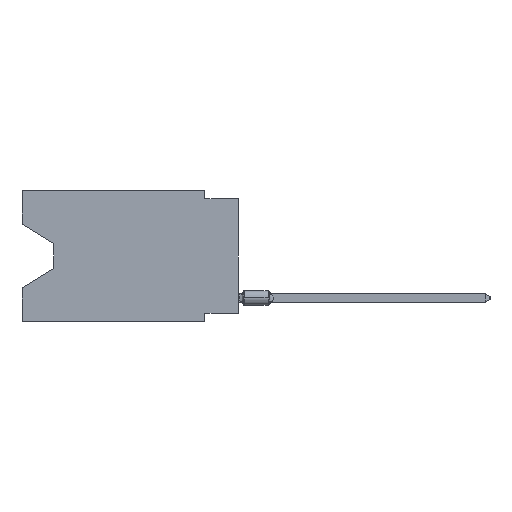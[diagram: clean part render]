
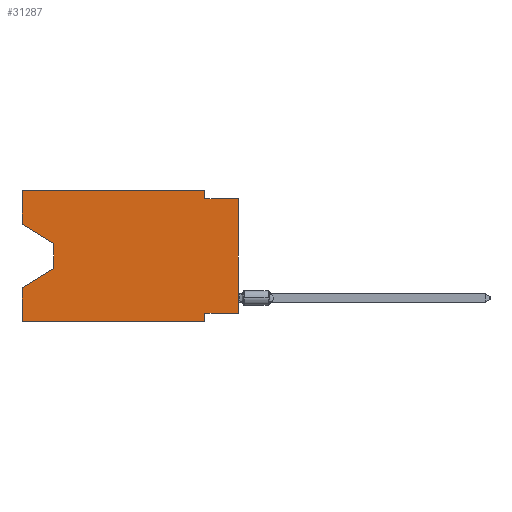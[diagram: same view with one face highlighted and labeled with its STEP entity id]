
A CAD part, left-side view. The second image highlights one B-rep face of the part: STEP entity #31287.
In plain terms, the highlighted planar face has unit normal (-1, 0, 0).
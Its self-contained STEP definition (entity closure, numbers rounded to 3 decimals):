
#125 = DIRECTION ( 'NONE',  ( 0., -1., 0. ) ) ;
#308 = LINE ( 'NONE', #8525, #14519 ) ;
#817 = EDGE_LOOP ( 'NONE', ( #17365, #26745, #19887, #10592, #1843, #28279, #2164, #14167, #22640, #7682, #24752, #28657 ) ) ;
#1843 = ORIENTED_EDGE ( 'NONE', *, *, #13814, .T. ) ;
#2164 = ORIENTED_EDGE ( 'NONE', *, *, #15014, .F. ) ;
#2192 = PLANE ( 'NONE',  #24027 ) ;
#2262 = DIRECTION ( 'NONE',  ( 0., 0.855, -0.519 ) ) ;
#2715 = CARTESIAN_POINT ( 'NONE',  ( 0., 16.383, -2.546 ) ) ;
#2917 = CARTESIAN_POINT ( 'NONE',  ( 0., 13.97, -4.013 ) ) ;
#3113 = VECTOR ( 'NONE', #27733, 1000. ) ;
#3210 = VERTEX_POINT ( 'NONE', #22563 ) ;
#3453 = DIRECTION ( 'NONE',  ( 0., 0., 1. ) ) ;
#4408 = DIRECTION ( 'NONE',  ( 1., 0., 0. ) ) ;
#4521 = CARTESIAN_POINT ( 'NONE',  ( 0., 2.54, -9.906 ) ) ;
#4547 = VERTEX_POINT ( 'NONE', #11504 ) ;
#6023 = VECTOR ( 'NONE', #19433, 1000. ) ;
#6717 = CARTESIAN_POINT ( 'NONE',  ( 0., 16.383, 0. ) ) ;
#7682 = ORIENTED_EDGE ( 'NONE', *, *, #28878, .F. ) ;
#7961 = CARTESIAN_POINT ( 'NONE',  ( 0., 16.383, -7.36 ) ) ;
#7990 = DIRECTION ( 'NONE',  ( 0., -1., 0. ) ) ;
#8167 = CARTESIAN_POINT ( 'NONE',  ( 0., 16.383, 0. ) ) ;
#8381 = LINE ( 'NONE', #19531, #22741 ) ;
#8525 = CARTESIAN_POINT ( 'NONE',  ( 0., 0., -0.635 ) ) ;
#8917 = DIRECTION ( 'NONE',  ( 0., 0., 1. ) ) ;
#10171 = LINE ( 'NONE', #21320, #15513 ) ;
#10301 = CARTESIAN_POINT ( 'NONE',  ( 0., 2.54, 0. ) ) ;
#10577 = DIRECTION ( 'NONE',  ( 0., 0., -1. ) ) ;
#10592 = ORIENTED_EDGE ( 'NONE', *, *, #18751, .F. ) ;
#10702 = DIRECTION ( 'NONE',  ( 0., 0., -1. ) ) ;
#11213 = LINE ( 'NONE', #4521, #6023 ) ;
#11255 = VERTEX_POINT ( 'NONE', #15968 ) ;
#11345 = CARTESIAN_POINT ( 'NONE',  ( 0., 0., -0.635 ) ) ;
#11444 = EDGE_CURVE ( 'NONE', #25396, #13808, #308, .T. ) ;
#11504 = CARTESIAN_POINT ( 'NONE',  ( 0., 13.97, -5.893 ) ) ;
#12002 = VECTOR ( 'NONE', #20411, 1000. ) ;
#13296 = EDGE_CURVE ( 'NONE', #3210, #30703, #11213, .T. ) ;
#13596 = LINE ( 'NONE', #27284, #18407 ) ;
#13808 = VERTEX_POINT ( 'NONE', #11345 ) ;
#13814 = EDGE_CURVE ( 'NONE', #27482, #30703, #17544, .T. ) ;
#14167 = ORIENTED_EDGE ( 'NONE', *, *, #35655, .T. ) ;
#14519 = VECTOR ( 'NONE', #125, 1000. ) ;
#14592 = LINE ( 'NONE', #15304, #20097 ) ;
#14639 = DIRECTION ( 'NONE',  ( 0., -1., 0. ) ) ;
#15014 = EDGE_CURVE ( 'NONE', #17722, #3210, #14592, .T. ) ;
#15304 = CARTESIAN_POINT ( 'NONE',  ( 0., 0., -9.271 ) ) ;
#15513 = VECTOR ( 'NONE', #10702, 1000. ) ;
#15968 = CARTESIAN_POINT ( 'NONE',  ( 0., 16.383, 0. ) ) ;
#16700 = CARTESIAN_POINT ( 'NONE',  ( 0., 13.97, -4.013 ) ) ;
#16781 = VECTOR ( 'NONE', #27947, 1000. ) ;
#16807 = VECTOR ( 'NONE', #7990, 1000. ) ;
#17365 = ORIENTED_EDGE ( 'NONE', *, *, #19311, .T. ) ;
#17544 = LINE ( 'NONE', #22486, #24815 ) ;
#17722 = VERTEX_POINT ( 'NONE', #20511 ) ;
#18407 = VECTOR ( 'NONE', #2262, 1000. ) ;
#18681 = EDGE_CURVE ( 'NONE', #4547, #27588, #13596, .T. ) ;
#18751 = EDGE_CURVE ( 'NONE', #27482, #27588, #23874, .T. ) ;
#19311 = EDGE_CURVE ( 'NONE', #30174, #34681, #22076, .T. ) ;
#19433 = DIRECTION ( 'NONE',  ( 0., 0., -1. ) ) ;
#19531 = CARTESIAN_POINT ( 'NONE',  ( 0., 0., 0. ) ) ;
#19887 = ORIENTED_EDGE ( 'NONE', *, *, #18681, .T. ) ;
#20024 = VECTOR ( 'NONE', #8917, 1000. ) ;
#20084 = VERTEX_POINT ( 'NONE', #10301 ) ;
#20097 = VECTOR ( 'NONE', #23164, 1000. ) ;
#20411 = DIRECTION ( 'NONE',  ( 0., 0., 1. ) ) ;
#20511 = CARTESIAN_POINT ( 'NONE',  ( 0., 0., -9.271 ) ) ;
#21212 = CARTESIAN_POINT ( 'NONE',  ( 0., 2.54, -0.635 ) ) ;
#21320 = CARTESIAN_POINT ( 'NONE',  ( 0., 2.54, 0. ) ) ;
#22076 = LINE ( 'NONE', #2715, #3113 ) ;
#22486 = CARTESIAN_POINT ( 'NONE',  ( 0., 16.383, -9.906 ) ) ;
#22563 = CARTESIAN_POINT ( 'NONE',  ( 0., 2.54, -9.271 ) ) ;
#22640 = ORIENTED_EDGE ( 'NONE', *, *, #11444, .F. ) ;
#22741 = VECTOR ( 'NONE', #3453, 1000. ) ;
#23164 = DIRECTION ( 'NONE',  ( 0., 1., 0. ) ) ;
#23874 = LINE ( 'NONE', #6717, #12002 ) ;
#24027 = AXIS2_PLACEMENT_3D ( 'NONE', #24465, #4408, #10577 ) ;
#24377 = EDGE_CURVE ( 'NONE', #34681, #4547, #25192, .T. ) ;
#24465 = CARTESIAN_POINT ( 'NONE',  ( 0., 16.383, 0. ) ) ;
#24690 = EDGE_CURVE ( 'NONE', #11255, #20084, #33199, .T. ) ;
#24752 = ORIENTED_EDGE ( 'NONE', *, *, #24690, .F. ) ;
#24815 = VECTOR ( 'NONE', #14639, 1000. ) ;
#25192 = LINE ( 'NONE', #2917, #16781 ) ;
#25396 = VERTEX_POINT ( 'NONE', #21212 ) ;
#26016 = CARTESIAN_POINT ( 'NONE',  ( 0., 2.54, -9.906 ) ) ;
#26745 = ORIENTED_EDGE ( 'NONE', *, *, #24377, .T. ) ;
#27219 = FACE_OUTER_BOUND ( 'NONE', #817, .T. ) ;
#27284 = CARTESIAN_POINT ( 'NONE',  ( 0., 13.97, -5.893 ) ) ;
#27382 = CARTESIAN_POINT ( 'NONE',  ( 0., 16.383, -2.546 ) ) ;
#27482 = VERTEX_POINT ( 'NONE', #35534 ) ;
#27588 = VERTEX_POINT ( 'NONE', #7961 ) ;
#27733 = DIRECTION ( 'NONE',  ( 0., -0.855, -0.519 ) ) ;
#27947 = DIRECTION ( 'NONE',  ( 0., 0., -1. ) ) ;
#28279 = ORIENTED_EDGE ( 'NONE', *, *, #13296, .F. ) ;
#28657 = ORIENTED_EDGE ( 'NONE', *, *, #32861, .F. ) ;
#28878 = EDGE_CURVE ( 'NONE', #20084, #25396, #10171, .T. ) ;
#30174 = VERTEX_POINT ( 'NONE', #27382 ) ;
#30703 = VERTEX_POINT ( 'NONE', #26016 ) ;
#31287 = ADVANCED_FACE ( 'NONE', ( #27219 ), #2192, .F. ) ;
#32861 = EDGE_CURVE ( 'NONE', #30174, #11255, #34116, .T. ) ;
#33199 = LINE ( 'NONE', #8167, #16807 ) ;
#34116 = LINE ( 'NONE', #34660, #20024 ) ;
#34660 = CARTESIAN_POINT ( 'NONE',  ( 0., 16.383, 0. ) ) ;
#34681 = VERTEX_POINT ( 'NONE', #16700 ) ;
#35534 = CARTESIAN_POINT ( 'NONE',  ( 0., 16.383, -9.906 ) ) ;
#35655 = EDGE_CURVE ( 'NONE', #17722, #13808, #8381, .T. ) ;
